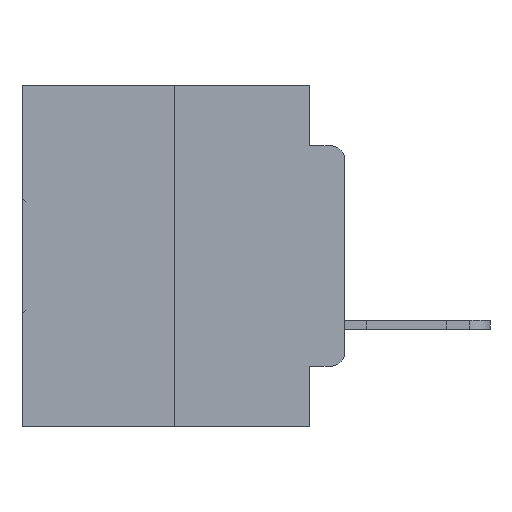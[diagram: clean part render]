
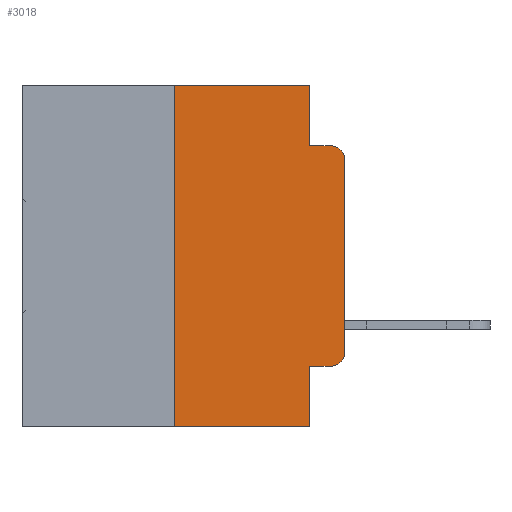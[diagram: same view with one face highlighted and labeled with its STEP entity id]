
A CAD part, left-side view. The second image highlights one B-rep face of the part: STEP entity #3018.
In plain terms, the highlighted planar face has unit normal (-1, 0, 0).
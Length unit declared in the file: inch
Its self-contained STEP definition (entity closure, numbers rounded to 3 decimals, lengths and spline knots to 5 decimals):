
#327 = LINE ( 'NONE', #3466, #24241 ) ;
#730 = EDGE_CURVE ( 'NONE', #9550, #16638, #8813, .T. ) ;
#900 = CARTESIAN_POINT ( 'NONE',  ( 0., 0.25, 0. ) ) ;
#2295 = DIRECTION ( 'NONE',  ( 0., 0., 1. ) ) ;
#2387 = CARTESIAN_POINT ( 'NONE',  ( 0., 0., -0.1085 ) ) ;
#2422 = VERTEX_POINT ( 'NONE', #12645 ) ;
#2660 = CARTESIAN_POINT ( 'NONE',  ( 0., 0.051, -0.0885 ) ) ;
#3018 = ADVANCED_FACE ( 'NONE', ( #25432 ), #24905, .F. ) ;
#3466 = CARTESIAN_POINT ( 'NONE',  ( 0., 0.051, -0.4115 ) ) ;
#3578 = DIRECTION ( 'NONE',  ( 0., -1., 0. ) ) ;
#3705 = VECTOR ( 'NONE', #22532, 39.37008 ) ;
#5069 = DIRECTION ( 'NONE',  ( -1., 0., 0. ) ) ;
#5219 = VECTOR ( 'NONE', #3578, 39.37008 ) ;
#5656 = CARTESIAN_POINT ( 'NONE',  ( 0., 0.25, 0. ) ) ;
#5883 = DIRECTION ( 'NONE',  ( -1., 0., 0. ) ) ;
#7454 = VERTEX_POINT ( 'NONE', #900 ) ;
#7705 = VERTEX_POINT ( 'NONE', #23179 ) ;
#8036 = CARTESIAN_POINT ( 'NONE',  ( 0., 0.051, 0. ) ) ;
#8046 = VECTOR ( 'NONE', #30649, 39.37008 ) ;
#8463 = VECTOR ( 'NONE', #2295, 39.37008 ) ;
#8671 = DIRECTION ( 'NONE',  ( 0., -1., 0. ) ) ;
#8813 = LINE ( 'NONE', #30518, #8046 ) ;
#8827 = CIRCLE ( 'NONE', #9291, 0.02 ) ;
#9291 = AXIS2_PLACEMENT_3D ( 'NONE', #20298, #5883, #22738 ) ;
#9550 = VERTEX_POINT ( 'NONE', #21331 ) ;
#9989 = AXIS2_PLACEMENT_3D ( 'NONE', #27633, #20090, #19862 ) ;
#10176 = DIRECTION ( 'NONE',  ( 0., 0., -1. ) ) ;
#10357 = VECTOR ( 'NONE', #29170, 39.37008 ) ;
#12263 = CARTESIAN_POINT ( 'NONE',  ( 0., 0.051, 0. ) ) ;
#12584 = CARTESIAN_POINT ( 'NONE',  ( 0., 0.051, 0. ) ) ;
#12645 = CARTESIAN_POINT ( 'NONE',  ( 0., 0.051, -0.0885 ) ) ;
#13133 = VERTEX_POINT ( 'NONE', #15212 ) ;
#13165 = EDGE_LOOP ( 'NONE', ( #22167, #22201, #22348, #22621, #22681, #22715, #23064, #23216, #23245, #23260 ) ) ;
#13413 = CARTESIAN_POINT ( 'NONE',  ( 0., 0.473, 0. ) ) ;
#14153 = VERTEX_POINT ( 'NONE', #14890 ) ;
#14665 = VERTEX_POINT ( 'NONE', #12263 ) ;
#14890 = CARTESIAN_POINT ( 'NONE',  ( 0., 0.02, -0.0885 ) ) ;
#15212 = CARTESIAN_POINT ( 'NONE',  ( 0., 0.051, -0.4115 ) ) ;
#15578 = CIRCLE ( 'NONE', #19525, 0.02 ) ;
#15684 = CARTESIAN_POINT ( 'NONE',  ( 0., 0.051, -0.5 ) ) ;
#16361 = EDGE_CURVE ( 'NONE', #7705, #29069, #27429, .T. ) ;
#16392 = EDGE_CURVE ( 'NONE', #29069, #14153, #15578, .T. ) ;
#16434 = EDGE_CURVE ( 'NONE', #14665, #2422, #31171, .T. ) ;
#16480 = EDGE_CURVE ( 'NONE', #2422, #14153, #18198, .T. ) ;
#16530 = EDGE_CURVE ( 'NONE', #13133, #16638, #29101, .T. ) ;
#16533 = EDGE_CURVE ( 'NONE', #9550, #7454, #22345, .T. ) ;
#16574 = EDGE_CURVE ( 'NONE', #18032, #7705, #8827, .T. ) ;
#16638 = VERTEX_POINT ( 'NONE', #15684 ) ;
#16659 = EDGE_CURVE ( 'NONE', #13133, #18032, #327, .T. ) ;
#18032 = VERTEX_POINT ( 'NONE', #27740 ) ;
#18198 = LINE ( 'NONE', #2660, #23881 ) ;
#18960 = VECTOR ( 'NONE', #10176, 39.37008 ) ;
#19483 = CARTESIAN_POINT ( 'NONE',  ( 0., 0., 0. ) ) ;
#19525 = AXIS2_PLACEMENT_3D ( 'NONE', #19594, #5069, #21997 ) ;
#19594 = CARTESIAN_POINT ( 'NONE',  ( 0., 0.02, -0.1085 ) ) ;
#19862 = DIRECTION ( 'NONE',  ( 0., 0., -1. ) ) ;
#20090 = DIRECTION ( 'NONE',  ( 1., 0., 0. ) ) ;
#20298 = CARTESIAN_POINT ( 'NONE',  ( 0., 0.02, -0.3915 ) ) ;
#21331 = CARTESIAN_POINT ( 'NONE',  ( 0., 0.25, -0.5 ) ) ;
#21997 = DIRECTION ( 'NONE',  ( 0., 0., -1. ) ) ;
#22167 = ORIENTED_EDGE ( 'NONE', *, *, #16361, .T. ) ;
#22201 = ORIENTED_EDGE ( 'NONE', *, *, #16392, .T. ) ;
#22345 = LINE ( 'NONE', #5656, #3705 ) ;
#22348 = ORIENTED_EDGE ( 'NONE', *, *, #16480, .F. ) ;
#22532 = DIRECTION ( 'NONE',  ( 0., 0., 1. ) ) ;
#22621 = ORIENTED_EDGE ( 'NONE', *, *, #16434, .F. ) ;
#22681 = ORIENTED_EDGE ( 'NONE', *, *, #23933, .F. ) ;
#22715 = ORIENTED_EDGE ( 'NONE', *, *, #16533, .F. ) ;
#22738 = DIRECTION ( 'NONE',  ( 0., 0., -1. ) ) ;
#23064 = ORIENTED_EDGE ( 'NONE', *, *, #730, .T. ) ;
#23179 = CARTESIAN_POINT ( 'NONE',  ( 0., 0., -0.3915 ) ) ;
#23216 = ORIENTED_EDGE ( 'NONE', *, *, #16530, .F. ) ;
#23245 = ORIENTED_EDGE ( 'NONE', *, *, #16659, .T. ) ;
#23260 = ORIENTED_EDGE ( 'NONE', *, *, #16574, .T. ) ;
#23881 = VECTOR ( 'NONE', #24740, 39.37008 ) ;
#23933 = EDGE_CURVE ( 'NONE', #7454, #14665, #30399, .T. ) ;
#24241 = VECTOR ( 'NONE', #8671, 39.37008 ) ;
#24740 = DIRECTION ( 'NONE',  ( 0., -1., 0. ) ) ;
#24905 = PLANE ( 'NONE',  #9989 ) ;
#25432 = FACE_OUTER_BOUND ( 'NONE', #13165, .T. ) ;
#27429 = LINE ( 'NONE', #19483, #8463 ) ;
#27633 = CARTESIAN_POINT ( 'NONE',  ( 0., 0.473, 0. ) ) ;
#27740 = CARTESIAN_POINT ( 'NONE',  ( 0., 0.02, -0.4115 ) ) ;
#29069 = VERTEX_POINT ( 'NONE', #2387 ) ;
#29101 = LINE ( 'NONE', #8036, #10357 ) ;
#29170 = DIRECTION ( 'NONE',  ( 0., 0., -1. ) ) ;
#30399 = LINE ( 'NONE', #13413, #5219 ) ;
#30518 = CARTESIAN_POINT ( 'NONE',  ( 0., 0.473, -0.5 ) ) ;
#30649 = DIRECTION ( 'NONE',  ( 0., -1., 0. ) ) ;
#31171 = LINE ( 'NONE', #12584, #18960 ) ;
